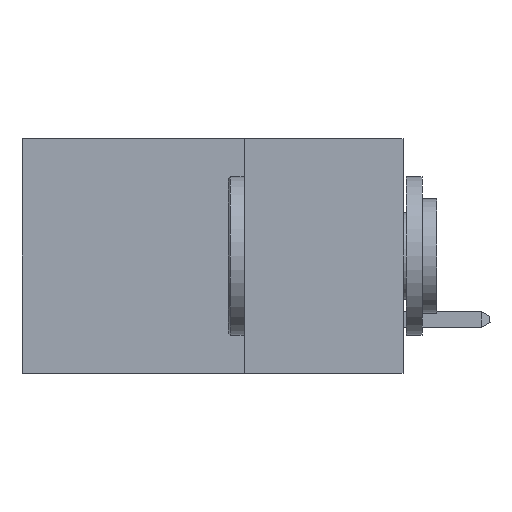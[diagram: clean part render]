
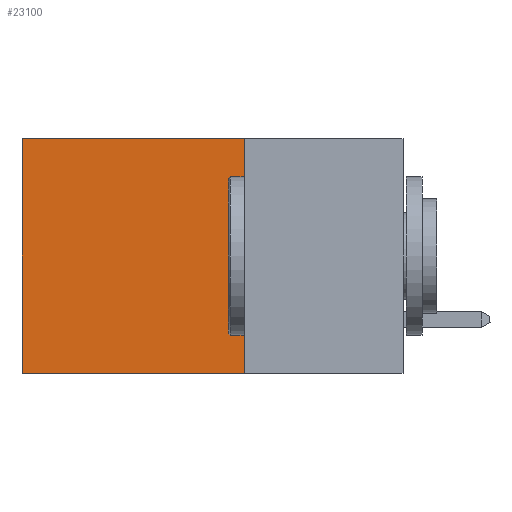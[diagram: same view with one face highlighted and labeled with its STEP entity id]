
A CAD part, left-side view. The second image highlights one B-rep face of the part: STEP entity #23100.
In plain terms, the highlighted planar face has unit normal (-1, 0, 0).
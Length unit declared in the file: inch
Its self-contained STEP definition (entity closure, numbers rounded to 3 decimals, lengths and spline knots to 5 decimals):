
#81 = VECTOR ( 'NONE', #3570, 39.37008 ) ;
#865 = VERTEX_POINT ( 'NONE', #40887 ) ;
#1293 = FACE_OUTER_BOUND ( 'NONE', #7542, .T. ) ;
#1393 = CARTESIAN_POINT ( 'NONE',  ( 0.2875, 0.25, 0. ) ) ;
#3570 = DIRECTION ( 'NONE',  ( 0., 1., 0. ) ) ;
#4355 = LINE ( 'NONE', #17377, #44260 ) ;
#6817 = VECTOR ( 'NONE', #11894, 39.37008 ) ;
#7542 = EDGE_LOOP ( 'NONE', ( #26012, #13838, #28211, #14330 ) ) ;
#8712 = EDGE_CURVE ( 'NONE', #36962, #865, #39527, .T. ) ;
#9497 = VERTEX_POINT ( 'NONE', #21034 ) ;
#9766 = CARTESIAN_POINT ( 'NONE',  ( 0.2875, 0.25, 0. ) ) ;
#11084 = VECTOR ( 'NONE', #26827, 39.37008 ) ;
#11894 = DIRECTION ( 'NONE',  ( 0., 0., -1. ) ) ;
#13838 = ORIENTED_EDGE ( 'NONE', *, *, #14669, .F. ) ;
#14330 = ORIENTED_EDGE ( 'NONE', *, *, #39968, .T. ) ;
#14669 = EDGE_CURVE ( 'NONE', #865, #40318, #45490, .T. ) ;
#14814 = EDGE_CURVE ( 'NONE', #9497, #40318, #41108, .T. ) ;
#17377 = CARTESIAN_POINT ( 'NONE',  ( 0.2875, 0.25, 0. ) ) ;
#20747 = DIRECTION ( 'NONE',  ( 0., 0., -1. ) ) ;
#21034 = CARTESIAN_POINT ( 'NONE',  ( 0.2875, 0.6, 0. ) ) ;
#23100 = ADVANCED_FACE ( 'NONE', ( #1293 ), #28552, .F. ) ;
#24717 = DIRECTION ( 'NONE',  ( 1., 0., 0. ) ) ;
#24735 = CARTESIAN_POINT ( 'NONE',  ( 0.2875, 0.25, -0.37 ) ) ;
#26012 = ORIENTED_EDGE ( 'NONE', *, *, #14814, .T. ) ;
#26827 = DIRECTION ( 'NONE',  ( 0., 0., -1. ) ) ;
#28211 = ORIENTED_EDGE ( 'NONE', *, *, #8712, .F. ) ;
#28552 = PLANE ( 'NONE',  #28892 ) ;
#28892 = AXIS2_PLACEMENT_3D ( 'NONE', #9766, #24717, #20747 ) ;
#30859 = CARTESIAN_POINT ( 'NONE',  ( 0.2875, 0.6, 0. ) ) ;
#31984 = CARTESIAN_POINT ( 'NONE',  ( 0.2875, 0.25, 0. ) ) ;
#33677 = CARTESIAN_POINT ( 'NONE',  ( 0.2875, 0.6, -0.37 ) ) ;
#36962 = VERTEX_POINT ( 'NONE', #31984 ) ;
#39527 = LINE ( 'NONE', #1393, #6817 ) ;
#39968 = EDGE_CURVE ( 'NONE', #36962, #9497, #4355, .T. ) ;
#40318 = VERTEX_POINT ( 'NONE', #33677 ) ;
#40887 = CARTESIAN_POINT ( 'NONE',  ( 0.2875, 0.25, -0.37 ) ) ;
#41108 = LINE ( 'NONE', #30859, #11084 ) ;
#41786 = DIRECTION ( 'NONE',  ( 0., 1., 0. ) ) ;
#44260 = VECTOR ( 'NONE', #41786, 39.37008 ) ;
#45490 = LINE ( 'NONE', #24735, #81 ) ;
